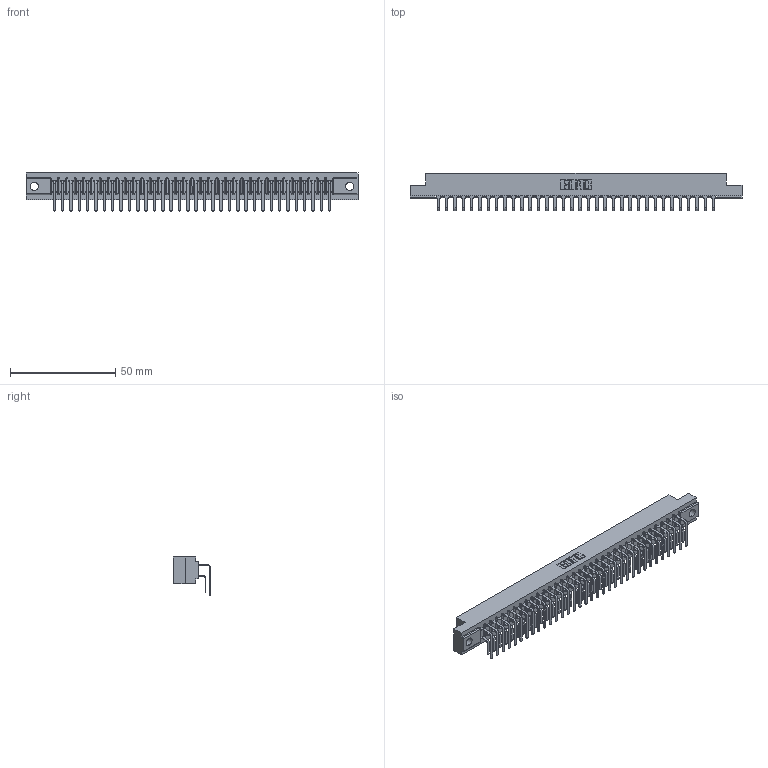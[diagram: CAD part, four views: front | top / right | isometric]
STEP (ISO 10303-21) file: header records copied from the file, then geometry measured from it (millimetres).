
FILE_DESCRIPTION (( 'STEP AP203' ), '1' );
FILE_NAME ('307-068-459-204.STEP', '2020-09-30T21:57:30', ( '' ), ( '' ), 'SwSTEP 2.0', 'SolidWorks 2020', '' );
FILE_SCHEMA (( 'CONFIG_CONTROL_DESIGN' ));
Length unit declared in the file: inch
Products named in the file (4): 307 Part_.156 Dia Mounting Holes; 307-068-459-204; 307-290-001_558 559 - 1 (Single); 307-290-001_559 - 2 (Single)
Assembly tree (69 placements, depth 2):
  307-068-459-204
    307 Part_.156 Dia Mounting Holes
    307-290-001_558 559 - 1 (Single)  x34
    307-290-001_559 - 2 (Single)  x34
Bounding box: 157.73 x 17.69 x 18.07 mm (x, y, z)
Volume: 16912 mm3; surface area: 22120.9 mm2
Topology: 69 solids, 69 shells, 3567 faces, 10015 edges, 6490 vertices
Faces by surface type: plane 2328, cylinder 1169, sphere 70
Entity records: 33087 total; most frequent: CARTESIAN_POINT 5422, ORIENTED_EDGE 5370, DIRECTION 5305, EDGE_CURVE 2685, LINE 2063, VECTOR 2063, VERTEX_POINT 1738, AXIS2_PLACEMENT_3D 1621
